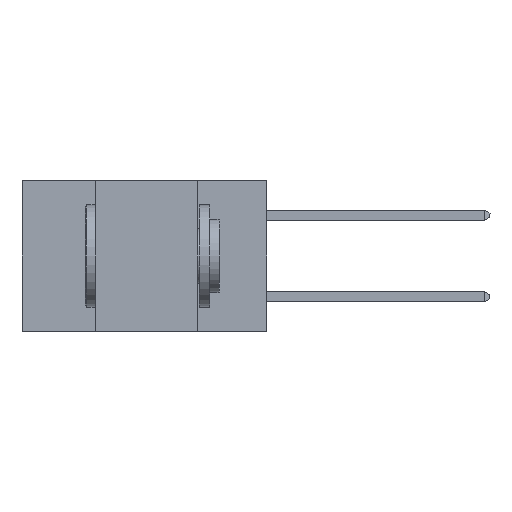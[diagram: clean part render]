
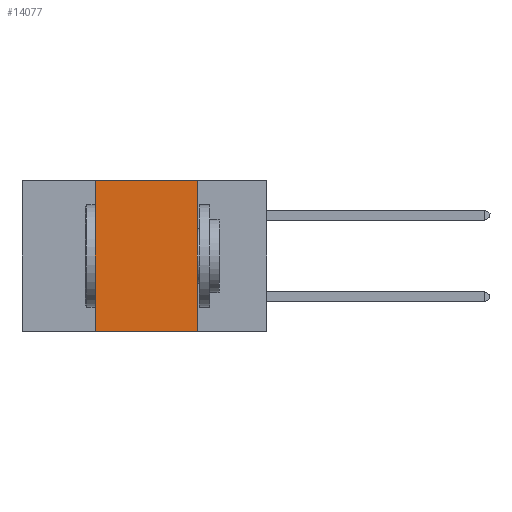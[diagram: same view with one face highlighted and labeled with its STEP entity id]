
A CAD part, left-side view. The second image highlights one B-rep face of the part: STEP entity #14077.
In plain terms, the highlighted planar face has unit normal (-1, 0, 0).
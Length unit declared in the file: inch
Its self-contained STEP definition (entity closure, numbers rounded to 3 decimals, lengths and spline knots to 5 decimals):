
#217 = EDGE_LOOP ( 'NONE', ( #10556, #10295, #10132, #11571 ) ) ;
#244 = EDGE_CURVE ( 'NONE', #1587, #8067, #5254, .T. ) ;
#499 = LINE ( 'NONE', #2042, #3052 ) ;
#1129 = CARTESIAN_POINT ( 'NONE',  ( 0., 0.6, -0.37 ) ) ;
#1320 = CARTESIAN_POINT ( 'NONE',  ( 0., 0.17, -0.37 ) ) ;
#1587 = VERTEX_POINT ( 'NONE', #5360 ) ;
#1856 = VERTEX_POINT ( 'NONE', #5974 ) ;
#2042 = CARTESIAN_POINT ( 'NONE',  ( 0., 0.42, 0. ) ) ;
#2217 = VERTEX_POINT ( 'NONE', #13320 ) ;
#2290 = CARTESIAN_POINT ( 'NONE',  ( 0., 0.6, 0. ) ) ;
#2625 = EDGE_CURVE ( 'NONE', #1856, #1587, #8855, .T. ) ;
#2840 = CARTESIAN_POINT ( 'NONE',  ( 0., 0.6, 0. ) ) ;
#3010 = AXIS2_PLACEMENT_3D ( 'NONE', #2290, #7802, #11251 ) ;
#3052 = VECTOR ( 'NONE', #9716, 39.37008 ) ;
#4427 = VECTOR ( 'NONE', #11236, 39.37008 ) ;
#5254 = LINE ( 'NONE', #13838, #11134 ) ;
#5360 = CARTESIAN_POINT ( 'NONE',  ( 0., 0.17, 0. ) ) ;
#5974 = CARTESIAN_POINT ( 'NONE',  ( 0., 0.42, 0. ) ) ;
#6814 = VECTOR ( 'NONE', #10528, 39.37008 ) ;
#7802 = DIRECTION ( 'NONE',  ( 1., 0., 0. ) ) ;
#8067 = VERTEX_POINT ( 'NONE', #1320 ) ;
#8855 = LINE ( 'NONE', #2840, #6814 ) ;
#9716 = DIRECTION ( 'NONE',  ( 0., 0., 1. ) ) ;
#10104 = LINE ( 'NONE', #1129, #4427 ) ;
#10132 = ORIENTED_EDGE ( 'NONE', *, *, #10836, .F. ) ;
#10295 = ORIENTED_EDGE ( 'NONE', *, *, #2625, .F. ) ;
#10375 = FACE_OUTER_BOUND ( 'NONE', #217, .T. ) ;
#10450 = EDGE_CURVE ( 'NONE', #2217, #8067, #10104, .T. ) ;
#10528 = DIRECTION ( 'NONE',  ( 0., -1., 0. ) ) ;
#10556 = ORIENTED_EDGE ( 'NONE', *, *, #244, .F. ) ;
#10836 = EDGE_CURVE ( 'NONE', #2217, #1856, #499, .T. ) ;
#11134 = VECTOR ( 'NONE', #12809, 39.37008 ) ;
#11236 = DIRECTION ( 'NONE',  ( 0., -1., 0. ) ) ;
#11251 = DIRECTION ( 'NONE',  ( 0., 0., -1. ) ) ;
#11571 = ORIENTED_EDGE ( 'NONE', *, *, #10450, .T. ) ;
#12809 = DIRECTION ( 'NONE',  ( 0., 0., -1. ) ) ;
#13320 = CARTESIAN_POINT ( 'NONE',  ( 0., 0.42, -0.37 ) ) ;
#13838 = CARTESIAN_POINT ( 'NONE',  ( 0., 0.17, 0. ) ) ;
#14077 = ADVANCED_FACE ( 'NONE', ( #10375 ), #14176, .F. ) ;
#14176 = PLANE ( 'NONE',  #3010 ) ;
